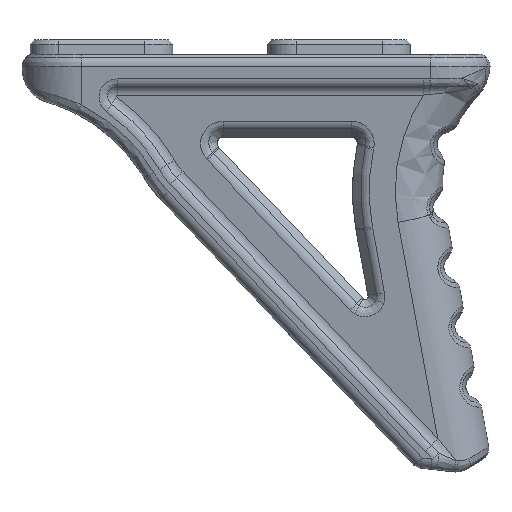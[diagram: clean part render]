
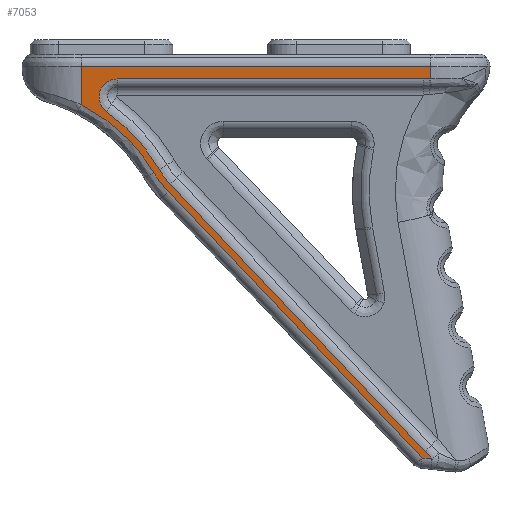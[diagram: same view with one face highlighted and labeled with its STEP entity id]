
A CAD part, left-side view. The second image highlights one B-rep face of the part: STEP entity #7053.
In plain terms, the highlighted planar face has unit normal (-0.99, 0, -0.139).
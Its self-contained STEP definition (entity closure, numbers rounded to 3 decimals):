
#68=PLANE('',#7528);
#147=ELLIPSE('',#7529,15.092,14.945);
#148=ELLIPSE('',#7530,9.088,9.);
#413=B_SPLINE_CURVE_WITH_KNOTS('',3,(#15262,#15263,#15264,#15265),
 .UNSPECIFIED.,.F.,.F.,(4,4),(-0.087,0.),.UNSPECIFIED.);
#414=B_SPLINE_CURVE_WITH_KNOTS('',3,(#15270,#15271,#15272,#15273),
 .UNSPECIFIED.,.F.,.F.,(4,4),(0.,0.156),.UNSPECIFIED.);
#415=B_SPLINE_CURVE_WITH_KNOTS('',3,(#15275,#15276,#15277,#15278),
 .UNSPECIFIED.,.F.,.F.,(4,4),(-0.668,0.),
 .UNSPECIFIED.);
#416=B_SPLINE_CURVE_WITH_KNOTS('',3,(#15280,#15281,#15282,#15283,#15284,
#15285,#15286),.UNSPECIFIED.,.F.,.F.,(4,1,1,1,4),(0.,0.083,
0.166,0.276,0.387),.UNSPECIFIED.);
#417=B_SPLINE_CURVE_WITH_KNOTS('',3,(#15290,#15291,#15292,#15293),
 .UNSPECIFIED.,.F.,.F.,(4,4),(-0.053,0.),.UNSPECIFIED.);
#418=B_SPLINE_CURVE_WITH_KNOTS('',3,(#15295,#15296,#15297,#15298),
 .UNSPECIFIED.,.F.,.F.,(4,4),(0.,0.007),.UNSPECIFIED.);
#1108=FACE_OUTER_BOUND('',#1575,.T.);
#1575=EDGE_LOOP('',(#5553,#5554,#5555,#5556,#5557,#5558,#5559,#5560,#5561,
#5562,#5563,#5564,#5565,#5566,#5567));
#1994=LINE('',#15157,#2333);
#1996=LINE('',#15268,#2335);
#1997=LINE('',#15288,#2336);
#1998=LINE('',#15300,#2337);
#1999=LINE('',#15302,#2338);
#2000=LINE('',#15304,#2339);
#2001=LINE('',#15309,#2340);
#2333=VECTOR('',#8362,10.);
#2335=VECTOR('',#8388,10.);
#2336=VECTOR('',#8389,10.);
#2337=VECTOR('',#8390,10.);
#2338=VECTOR('',#8391,10.);
#2339=VECTOR('',#8392,10.);
#2340=VECTOR('',#8397,10.);
#3118=VERTEX_POINT('',#15153);
#3120=VERTEX_POINT('',#15156);
#3124=VERTEX_POINT('',#15260);
#3125=VERTEX_POINT('',#15267);
#3126=VERTEX_POINT('',#15269);
#3127=VERTEX_POINT('',#15274);
#3128=VERTEX_POINT('',#15279);
#3129=VERTEX_POINT('',#15287);
#3130=VERTEX_POINT('',#15289);
#3131=VERTEX_POINT('',#15294);
#3132=VERTEX_POINT('',#15299);
#3133=VERTEX_POINT('',#15301);
#3134=VERTEX_POINT('',#15303);
#3135=VERTEX_POINT('',#15305);
#3136=VERTEX_POINT('',#15307);
#3962=EDGE_CURVE('',#3120,#3118,#1994,.T.);
#3975=EDGE_CURVE('',#3118,#3124,#413,.T.);
#3976=EDGE_CURVE('',#3124,#3125,#1996,.T.);
#3977=EDGE_CURVE('',#3125,#3126,#414,.T.);
#3978=EDGE_CURVE('',#3126,#3127,#415,.T.);
#3979=EDGE_CURVE('',#3127,#3128,#416,.T.);
#3980=EDGE_CURVE('',#3128,#3129,#1997,.T.);
#3981=EDGE_CURVE('',#3129,#3130,#417,.T.);
#3982=EDGE_CURVE('',#3130,#3131,#418,.T.);
#3983=EDGE_CURVE('',#3131,#3132,#1998,.T.);
#3984=EDGE_CURVE('',#3132,#3133,#1999,.T.);
#3985=EDGE_CURVE('',#3133,#3134,#2000,.T.);
#3986=EDGE_CURVE('',#3134,#3135,#147,.T.);
#3987=EDGE_CURVE('',#3135,#3136,#148,.T.);
#3988=EDGE_CURVE('',#3136,#3120,#2001,.T.);
#5553=ORIENTED_EDGE('',*,*,#3962,.T.);
#5554=ORIENTED_EDGE('',*,*,#3975,.T.);
#5555=ORIENTED_EDGE('',*,*,#3976,.T.);
#5556=ORIENTED_EDGE('',*,*,#3977,.T.);
#5557=ORIENTED_EDGE('',*,*,#3978,.T.);
#5558=ORIENTED_EDGE('',*,*,#3979,.T.);
#5559=ORIENTED_EDGE('',*,*,#3980,.T.);
#5560=ORIENTED_EDGE('',*,*,#3981,.T.);
#5561=ORIENTED_EDGE('',*,*,#3982,.T.);
#5562=ORIENTED_EDGE('',*,*,#3983,.T.);
#5563=ORIENTED_EDGE('',*,*,#3984,.T.);
#5564=ORIENTED_EDGE('',*,*,#3985,.T.);
#5565=ORIENTED_EDGE('',*,*,#3986,.T.);
#5566=ORIENTED_EDGE('',*,*,#3987,.T.);
#5567=ORIENTED_EDGE('',*,*,#3988,.T.);
#7053=ADVANCED_FACE('',(#1108),#68,.F.);
#7528=AXIS2_PLACEMENT_3D('',#15266,#8386,#8387);
#7529=AXIS2_PLACEMENT_3D('',#15306,#8393,#8394);
#7530=AXIS2_PLACEMENT_3D('',#15308,#8395,#8396);
#8362=DIRECTION('',(0.016,-0.993,-0.114));
#8386=DIRECTION('center_axis',(0.99,0.,0.139));
#8387=DIRECTION('ref_axis',(0.,-1.,0.));
#8388=DIRECTION('',(-0.101,0.686,0.72));
#8389=DIRECTION('',(0.,-1.,0.));
#8390=DIRECTION('',(-0.139,0.,0.99));
#8391=DIRECTION('',(0.,1.,0.));
#8392=DIRECTION('',(0.139,0.,-0.99));
#8393=DIRECTION('center_axis',(0.99,0.,0.139));
#8394=DIRECTION('ref_axis',(-0.139,0.,0.99));
#8395=DIRECTION('center_axis',(-0.99,0.,
-0.139));
#8396=DIRECTION('ref_axis',(0.139,0.,-0.99));
#8397=DIRECTION('',(0.101,-0.686,-0.72));
#15153=CARTESIAN_POINT('',(-7.71,-73.826,-36.882));
#15156=CARTESIAN_POINT('',(-7.724,-72.961,-36.783));
#15157=CARTESIAN_POINT('',(-8.027,-54.135,-34.627));
#15260=CARTESIAN_POINT('',(-7.8,-73.236,-36.244));
#15262=CARTESIAN_POINT('Ctrl Pts',(-7.71,-73.826,
-36.882));
#15263=CARTESIAN_POINT('Ctrl Pts',(-7.74,-73.633,-36.666));
#15264=CARTESIAN_POINT('Ctrl Pts',(-7.77,-73.436,-36.454));
#15265=CARTESIAN_POINT('Ctrl Pts',(-7.8,-73.236,
-36.244));
#15266=CARTESIAN_POINT('Origin',(-12.5,-37.3,-2.8));
#15267=CARTESIAN_POINT('',(-10.961,-51.798,-13.748));
#15268=CARTESIAN_POINT('',(-11.918,-45.308,-6.938));
#15269=CARTESIAN_POINT('',(-11.135,-50.872,-12.512));
#15270=CARTESIAN_POINT('Ctrl Pts',(-10.961,-51.798,
-13.748));
#15271=CARTESIAN_POINT('Ctrl Pts',(-11.014,-51.442,
-13.374));
#15272=CARTESIAN_POINT('Ctrl Pts',(-11.072,-51.13,
-12.958));
#15273=CARTESIAN_POINT('Ctrl Pts',(-11.135,-50.872,
-12.512));
#15274=CARTESIAN_POINT('',(-11.82,-46.429,-7.641));
#15275=CARTESIAN_POINT('Ctrl Pts',(-11.135,-50.872,
-12.512));
#15276=CARTESIAN_POINT('Ctrl Pts',(-11.404,-49.766,-10.598));
#15277=CARTESIAN_POINT('Ctrl Pts',(-11.639,-48.241,-8.923));
#15278=CARTESIAN_POINT('Ctrl Pts',(-11.82,-46.429,
-7.641));
#15279=CARTESIAN_POINT('',(-12.208,-47.314,-4.878));
#15280=CARTESIAN_POINT('Ctrl Pts',(-11.82,-46.429,
-7.641));
#15281=CARTESIAN_POINT('Ctrl Pts',(-11.842,-46.205,
-7.482));
#15282=CARTESIAN_POINT('Ctrl Pts',(-11.904,-45.845,
-7.04));
#15283=CARTESIAN_POINT('Ctrl Pts',(-12.036,-45.709,
-6.104));
#15284=CARTESIAN_POINT('Ctrl Pts',(-12.169,-46.21,
-5.157));
#15285=CARTESIAN_POINT('Ctrl Pts',(-12.208,-46.945,-4.878));
#15286=CARTESIAN_POINT('Ctrl Pts',(-12.208,-47.314,-4.878));
#15287=CARTESIAN_POINT('',(-12.208,-73.096,-4.878));
#15288=CARTESIAN_POINT('',(-12.208,-58.,-4.878));
#15289=CARTESIAN_POINT('',(-12.21,-73.63,-4.866));
#15290=CARTESIAN_POINT('Ctrl Pts',(-12.208,-73.096,-4.878));
#15291=CARTESIAN_POINT('Ctrl Pts',(-12.208,-73.274,-4.878));
#15292=CARTESIAN_POINT('Ctrl Pts',(-12.209,-73.452,
-4.874));
#15293=CARTESIAN_POINT('Ctrl Pts',(-12.21,-73.63,
-4.866));
#15294=CARTESIAN_POINT('',(-12.21,-73.7,-4.862));
#15295=CARTESIAN_POINT('Ctrl Pts',(-12.21,-73.63,
-4.866));
#15296=CARTESIAN_POINT('Ctrl Pts',(-12.21,-73.654,
-4.864));
#15297=CARTESIAN_POINT('Ctrl Pts',(-12.21,-73.677,
-4.863));
#15298=CARTESIAN_POINT('Ctrl Pts',(-12.21,-73.7,
-4.862));
#15299=CARTESIAN_POINT('',(-12.353,-73.7,-3.845));
#15300=CARTESIAN_POINT('',(-12.5,-73.7,-2.8));
#15301=CARTESIAN_POINT('',(-12.353,-44.3,-3.845));
#15302=CARTESIAN_POINT('',(-12.353,-42.3,-3.845));
#15303=CARTESIAN_POINT('',(-11.903,-44.3,-7.05));
#15304=CARTESIAN_POINT('',(-12.258,-44.3,-4.523));
#15305=CARTESIAN_POINT('',(-11.1,-50.387,-12.761));
#15306=CARTESIAN_POINT('Origin',(-10.031,-37.525,-20.37));
#15307=CARTESIAN_POINT('',(-10.871,-51.618,-14.388));
#15308=CARTESIAN_POINT('Origin',(-11.744,-58.134,-8.179));
#15309=CARTESIAN_POINT('',(-10.153,-56.488,-19.497));
